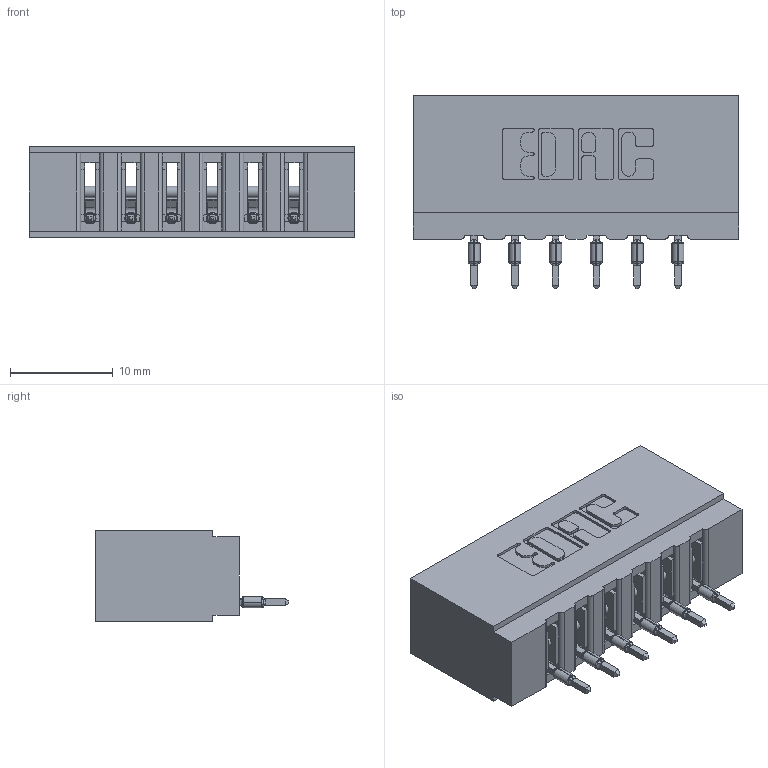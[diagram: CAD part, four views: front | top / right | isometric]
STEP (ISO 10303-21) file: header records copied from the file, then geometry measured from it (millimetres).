
FILE_DESCRIPTION (( 'STEP AP203' ), '1' );
FILE_NAME ('717-006-560-106.STEP', '2020-03-13T17:40:13', ( '' ), ( '' ), 'SwSTEP 2.0', 'SolidWorks 2016', '' );
FILE_SCHEMA (( 'CONFIG_CONTROL_DESIGN' ));
Length unit declared in the file: inch
Products named in the file (3): 717 Part_Insulator Option - 06; 745-292-001_560; 717-006-560-106
Assembly tree (7 placements, depth 2):
  717-006-560-106
    717 Part_Insulator Option - 06
    745-292-001_560  x6
Bounding box: 31.65 x 18.78 x 8.89 mm (x, y, z)
Volume: 2854.6 mm3; surface area: 3715.4 mm2
Topology: 7 solids, 7 shells, 826 faces, 2291 edges, 1462 vertices
Faces by surface type: plane 492, cylinder 178, bspline 120, torus 36
Entity records: 15282 total; most frequent: CARTESIAN_POINT 3193, ORIENTED_EDGE 2562, DIRECTION 2263, EDGE_CURVE 1281, VECTOR 1055, LINE 1055, VERTEX_POINT 822, AXIS2_PLACEMENT_3D 604
